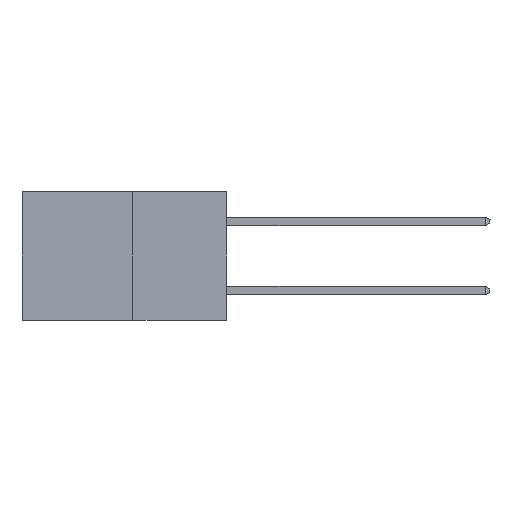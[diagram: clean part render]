
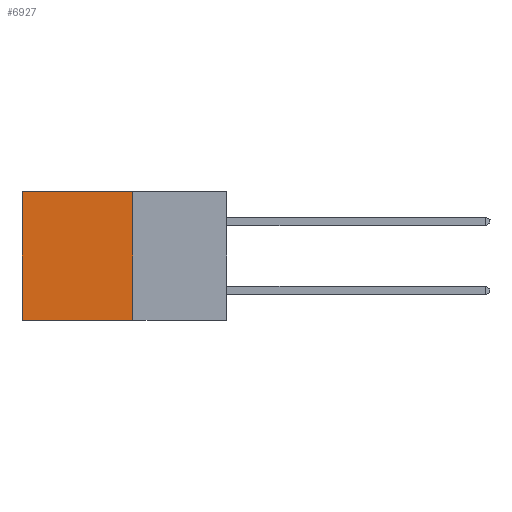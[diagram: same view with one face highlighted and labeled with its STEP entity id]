
A CAD part, left-side view. The second image highlights one B-rep face of the part: STEP entity #6927.
In plain terms, the highlighted planar face has unit normal (-1, 0, 0).
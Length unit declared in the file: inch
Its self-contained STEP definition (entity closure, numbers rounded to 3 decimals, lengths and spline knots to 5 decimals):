
#21 = VERTEX_POINT ( 'NONE', #3289 ) ;
#679 = EDGE_LOOP ( 'NONE', ( #2986, #2808, #2689, #2660 ) ) ;
#879 = LINE ( 'NONE', #3018, #6734 ) ;
#1330 = VERTEX_POINT ( 'NONE', #9070 ) ;
#1345 = DIRECTION ( 'NONE',  ( 0., 0., -1. ) ) ;
#2650 = VECTOR ( 'NONE', #1345, 39.37008 ) ;
#2660 = ORIENTED_EDGE ( 'NONE', *, *, #2967, .T. ) ;
#2675 = DIRECTION ( 'NONE',  ( 0., 0., -1. ) ) ;
#2689 = ORIENTED_EDGE ( 'NONE', *, *, #3940, .F. ) ;
#2808 = ORIENTED_EDGE ( 'NONE', *, *, #6682, .F. ) ;
#2967 = EDGE_CURVE ( 'NONE', #1330, #4293, #879, .T. ) ;
#2986 = ORIENTED_EDGE ( 'NONE', *, *, #9121, .T. ) ;
#3018 = CARTESIAN_POINT ( 'NONE',  ( 0.277, 0.27, 0. ) ) ;
#3289 = CARTESIAN_POINT ( 'NONE',  ( 0.277, 0.59, -0.37 ) ) ;
#3339 = VECTOR ( 'NONE', #7221, 39.37008 ) ;
#3521 = CARTESIAN_POINT ( 'NONE',  ( 0.277, 0.27, -0.37 ) ) ;
#3940 = EDGE_CURVE ( 'NONE', #1330, #5586, #4731, .T. ) ;
#4293 = VERTEX_POINT ( 'NONE', #8908 ) ;
#4731 = LINE ( 'NONE', #3521, #2650 ) ;
#5155 = DIRECTION ( 'NONE',  ( 0., 0., -1. ) ) ;
#5187 = DIRECTION ( 'NONE',  ( 1., 0., 0. ) ) ;
#5233 = CARTESIAN_POINT ( 'NONE',  ( 0.277, 0.27, -0.37 ) ) ;
#5237 = LINE ( 'NONE', #6507, #9132 ) ;
#5484 = PLANE ( 'NONE',  #9635 ) ;
#5586 = VERTEX_POINT ( 'NONE', #8484 ) ;
#6070 = DIRECTION ( 'NONE',  ( 0., 1., 0. ) ) ;
#6507 = CARTESIAN_POINT ( 'NONE',  ( 0.277, 0.59, -0.37 ) ) ;
#6682 = EDGE_CURVE ( 'NONE', #5586, #21, #7590, .T. ) ;
#6734 = VECTOR ( 'NONE', #6070, 39.37008 ) ;
#6927 = ADVANCED_FACE ( 'NONE', ( #9392 ), #5484, .F. ) ;
#7221 = DIRECTION ( 'NONE',  ( 0., 1., 0. ) ) ;
#7257 = CARTESIAN_POINT ( 'NONE',  ( 0.277, 0.27, -0.37 ) ) ;
#7590 = LINE ( 'NONE', #7257, #3339 ) ;
#8484 = CARTESIAN_POINT ( 'NONE',  ( 0.277, 0.27, -0.37 ) ) ;
#8908 = CARTESIAN_POINT ( 'NONE',  ( 0.277, 0.59, 0. ) ) ;
#9070 = CARTESIAN_POINT ( 'NONE',  ( 0.277, 0.27, 0. ) ) ;
#9121 = EDGE_CURVE ( 'NONE', #4293, #21, #5237, .T. ) ;
#9132 = VECTOR ( 'NONE', #2675, 39.37008 ) ;
#9392 = FACE_OUTER_BOUND ( 'NONE', #679, .T. ) ;
#9635 = AXIS2_PLACEMENT_3D ( 'NONE', #5233, #5187, #5155 ) ;
